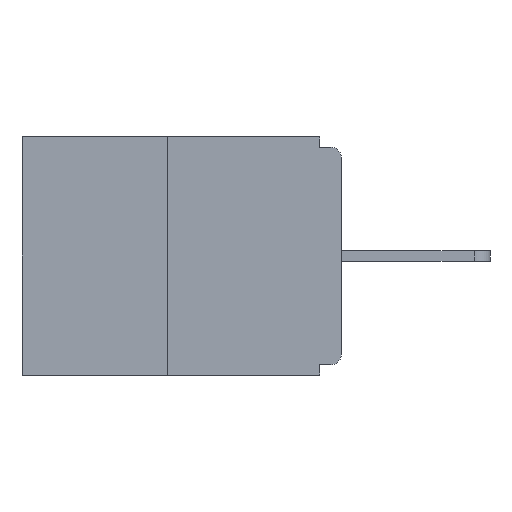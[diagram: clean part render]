
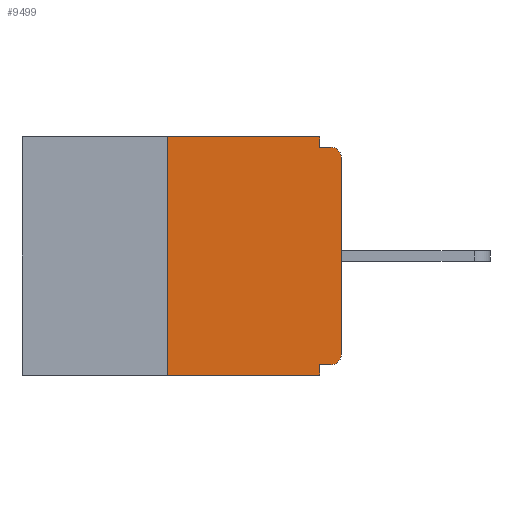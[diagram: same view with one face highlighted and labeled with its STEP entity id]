
A CAD part, left-side view. The second image highlights one B-rep face of the part: STEP entity #9499.
In plain terms, the highlighted planar face has unit normal (-1, 0, 0).
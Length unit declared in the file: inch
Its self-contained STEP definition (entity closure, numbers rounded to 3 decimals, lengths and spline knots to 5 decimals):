
#53 = VECTOR ( 'NONE', #7992, 39.37008 ) ;
#96 = LINE ( 'NONE', #1660, #18272 ) ;
#528 = ORIENTED_EDGE ( 'NONE', *, *, #5092, .F. ) ;
#1016 = DIRECTION ( 'NONE',  ( 0., -1., 0. ) ) ;
#1339 = FACE_OUTER_BOUND ( 'NONE', #7541, .T. ) ;
#1357 = VECTOR ( 'NONE', #21987, 39.37008 ) ;
#1646 = VERTEX_POINT ( 'NONE', #19557 ) ;
#1660 = CARTESIAN_POINT ( 'NONE',  ( 0., 0.46, -0.343 ) ) ;
#1676 = EDGE_CURVE ( 'NONE', #13311, #17903, #3189, .T. ) ;
#1785 = EDGE_CURVE ( 'NONE', #20814, #20795, #22539, .T. ) ;
#2222 = ORIENTED_EDGE ( 'NONE', *, *, #18852, .F. ) ;
#2257 = CARTESIAN_POINT ( 'NONE',  ( 0., 0., -0.03 ) ) ;
#2910 = LINE ( 'NONE', #17034, #7027 ) ;
#2930 = DIRECTION ( 'NONE',  ( 0., 0., -1. ) ) ;
#3189 = CIRCLE ( 'NONE', #8065, 0.015 ) ;
#3503 = VECTOR ( 'NONE', #7058, 39.37008 ) ;
#3637 = CARTESIAN_POINT ( 'NONE',  ( 0., 0., -0.313 ) ) ;
#3922 = CARTESIAN_POINT ( 'NONE',  ( 0., 0.015, -0.015 ) ) ;
#4178 = VERTEX_POINT ( 'NONE', #14351 ) ;
#4461 = EDGE_CURVE ( 'NONE', #22204, #20795, #9274, .T. ) ;
#5001 = ORIENTED_EDGE ( 'NONE', *, *, #21774, .F. ) ;
#5092 = EDGE_CURVE ( 'NONE', #4178, #7923, #11718, .T. ) ;
#6518 = EDGE_CURVE ( 'NONE', #17903, #20814, #16587, .T. ) ;
#6903 = ORIENTED_EDGE ( 'NONE', *, *, #1676, .T. ) ;
#7027 = VECTOR ( 'NONE', #10059, 39.37008 ) ;
#7058 = DIRECTION ( 'NONE',  ( 0., 0., -1. ) ) ;
#7541 = EDGE_LOOP ( 'NONE', ( #528, #10476, #15147, #15694, #2222, #6903, #16803, #21352, #8563, #5001 ) ) ;
#7923 = VERTEX_POINT ( 'NONE', #19038 ) ;
#7992 = DIRECTION ( 'NONE',  ( 0., 0., 1. ) ) ;
#8031 = LINE ( 'NONE', #13477, #16269 ) ;
#8065 = AXIS2_PLACEMENT_3D ( 'NONE', #18998, #18874, #18823 ) ;
#8197 = LINE ( 'NONE', #10519, #3503 ) ;
#8393 = EDGE_CURVE ( 'NONE', #19806, #10417, #20008, .T. ) ;
#8563 = ORIENTED_EDGE ( 'NONE', *, *, #4461, .F. ) ;
#8669 = DIRECTION ( 'NONE',  ( 0., -1., 0. ) ) ;
#9121 = CARTESIAN_POINT ( 'NONE',  ( 0., 0.031, -0.328 ) ) ;
#9256 = AXIS2_PLACEMENT_3D ( 'NONE', #18135, #14469, #14571 ) ;
#9274 = LINE ( 'NONE', #13372, #18594 ) ;
#9499 = ADVANCED_FACE ( 'NONE', ( #1339 ), #9919, .F. ) ;
#9919 = PLANE ( 'NONE',  #22025 ) ;
#10001 = DIRECTION ( 'NONE',  ( 0., 1., 0. ) ) ;
#10059 = DIRECTION ( 'NONE',  ( 0., 0., 1. ) ) ;
#10399 = CARTESIAN_POINT ( 'NONE',  ( 0., 0.015, -0.328 ) ) ;
#10417 = VERTEX_POINT ( 'NONE', #21440 ) ;
#10476 = ORIENTED_EDGE ( 'NONE', *, *, #17128, .F. ) ;
#10519 = CARTESIAN_POINT ( 'NONE',  ( 0., 0.031, 0. ) ) ;
#11525 = CARTESIAN_POINT ( 'NONE',  ( 0., 0., 0. ) ) ;
#11598 = CARTESIAN_POINT ( 'NONE',  ( 0., 0.031, -0.343 ) ) ;
#11679 = CARTESIAN_POINT ( 'NONE',  ( 0., 0.46, 0. ) ) ;
#11718 = LINE ( 'NONE', #13420, #19900 ) ;
#11805 = CARTESIAN_POINT ( 'NONE',  ( 0., 0.031, -0.015 ) ) ;
#13311 = VERTEX_POINT ( 'NONE', #10399 ) ;
#13372 = CARTESIAN_POINT ( 'NONE',  ( 0., 0., -0.015 ) ) ;
#13420 = CARTESIAN_POINT ( 'NONE',  ( 0., 0.46, 0. ) ) ;
#13475 = DIRECTION ( 'NONE',  ( 1., 0., 0. ) ) ;
#13477 = CARTESIAN_POINT ( 'NONE',  ( 0., 0., -0.328 ) ) ;
#14351 = CARTESIAN_POINT ( 'NONE',  ( 0., 0.25, 0. ) ) ;
#14469 = DIRECTION ( 'NONE',  ( -1., 0., 0. ) ) ;
#14571 = DIRECTION ( 'NONE',  ( 0., 0., -1. ) ) ;
#15147 = ORIENTED_EDGE ( 'NONE', *, *, #17266, .T. ) ;
#15694 = ORIENTED_EDGE ( 'NONE', *, *, #8393, .F. ) ;
#16269 = VECTOR ( 'NONE', #10001, 39.37008 ) ;
#16587 = LINE ( 'NONE', #11525, #53 ) ;
#16803 = ORIENTED_EDGE ( 'NONE', *, *, #6518, .T. ) ;
#17034 = CARTESIAN_POINT ( 'NONE',  ( 0., 0.25, 0. ) ) ;
#17128 = EDGE_CURVE ( 'NONE', #1646, #4178, #2910, .T. ) ;
#17266 = EDGE_CURVE ( 'NONE', #1646, #10417, #96, .T. ) ;
#17903 = VERTEX_POINT ( 'NONE', #3637 ) ;
#18135 = CARTESIAN_POINT ( 'NONE',  ( 0., 0.015, -0.03 ) ) ;
#18272 = VECTOR ( 'NONE', #8669, 39.37008 ) ;
#18594 = VECTOR ( 'NONE', #1016, 39.37008 ) ;
#18823 = DIRECTION ( 'NONE',  ( 0., 0., -1. ) ) ;
#18852 = EDGE_CURVE ( 'NONE', #13311, #19806, #8031, .T. ) ;
#18874 = DIRECTION ( 'NONE',  ( -1., 0., 0. ) ) ;
#18998 = CARTESIAN_POINT ( 'NONE',  ( 0., 0.015, -0.313 ) ) ;
#19038 = CARTESIAN_POINT ( 'NONE',  ( 0., 0.031, 0. ) ) ;
#19557 = CARTESIAN_POINT ( 'NONE',  ( 0., 0.25, -0.343 ) ) ;
#19806 = VERTEX_POINT ( 'NONE', #9121 ) ;
#19900 = VECTOR ( 'NONE', #20304, 39.37008 ) ;
#20008 = LINE ( 'NONE', #11598, #1357 ) ;
#20304 = DIRECTION ( 'NONE',  ( 0., -1., 0. ) ) ;
#20795 = VERTEX_POINT ( 'NONE', #3922 ) ;
#20814 = VERTEX_POINT ( 'NONE', #2257 ) ;
#21352 = ORIENTED_EDGE ( 'NONE', *, *, #1785, .T. ) ;
#21440 = CARTESIAN_POINT ( 'NONE',  ( 0., 0.031, -0.343 ) ) ;
#21774 = EDGE_CURVE ( 'NONE', #7923, #22204, #8197, .T. ) ;
#21987 = DIRECTION ( 'NONE',  ( 0., 0., -1. ) ) ;
#22025 = AXIS2_PLACEMENT_3D ( 'NONE', #11679, #13475, #2930 ) ;
#22204 = VERTEX_POINT ( 'NONE', #11805 ) ;
#22539 = CIRCLE ( 'NONE', #9256, 0.015 ) ;
